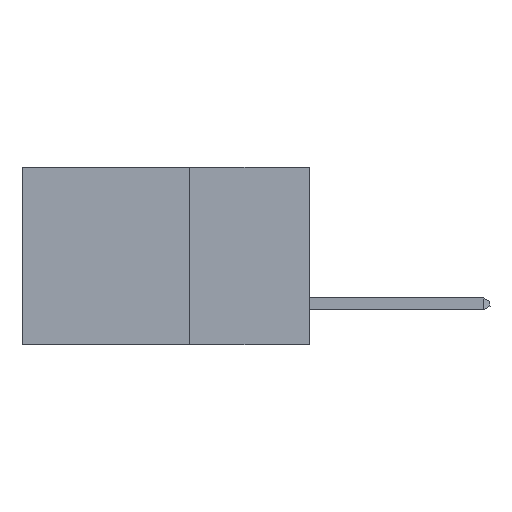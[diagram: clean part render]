
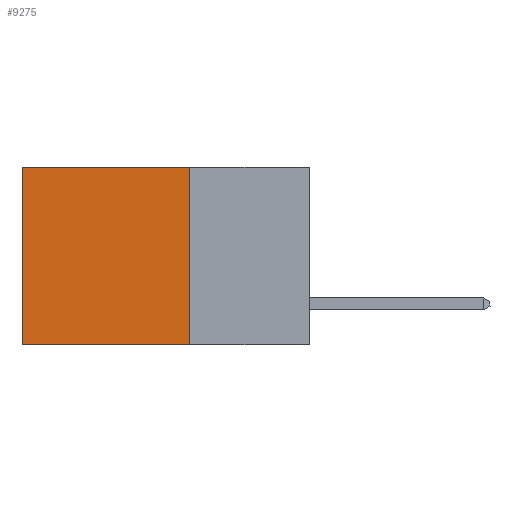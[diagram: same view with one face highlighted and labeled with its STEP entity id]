
A CAD part, left-side view. The second image highlights one B-rep face of the part: STEP entity #9275.
In plain terms, the highlighted planar face has unit normal (-1, 0, 0).
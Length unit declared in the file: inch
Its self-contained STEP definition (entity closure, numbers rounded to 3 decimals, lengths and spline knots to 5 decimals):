
#503 = EDGE_CURVE ( 'NONE', #8595, #10421, #12029, .T. ) ;
#1007 = EDGE_CURVE ( 'NONE', #14012, #10421, #18827, .T. ) ;
#1427 = CARTESIAN_POINT ( 'NONE',  ( 0.2875, 0.25, 0. ) ) ;
#1593 = EDGE_LOOP ( 'NONE', ( #12755, #6586, #19972, #16790 ) ) ;
#2520 = DIRECTION ( 'NONE',  ( 0., 1., 0. ) ) ;
#3064 = DIRECTION ( 'NONE',  ( 0., 0., -1. ) ) ;
#4185 = CARTESIAN_POINT ( 'NONE',  ( 0.2875, 0.6, -0.37 ) ) ;
#4750 = CARTESIAN_POINT ( 'NONE',  ( 0.2875, 0.25, 0. ) ) ;
#5290 = EDGE_CURVE ( 'NONE', #9811, #8595, #15781, .T. ) ;
#6255 = CARTESIAN_POINT ( 'NONE',  ( 0.2875, 0.25, -0.37 ) ) ;
#6586 = ORIENTED_EDGE ( 'NONE', *, *, #503, .F. ) ;
#7901 = PLANE ( 'NONE',  #13370 ) ;
#8172 = DIRECTION ( 'NONE',  ( 0., 0., -1. ) ) ;
#8595 = VERTEX_POINT ( 'NONE', #16961 ) ;
#9275 = ADVANCED_FACE ( 'NONE', ( #17598 ), #7901, .F. ) ;
#9811 = VERTEX_POINT ( 'NONE', #12326 ) ;
#10421 = VERTEX_POINT ( 'NONE', #4185 ) ;
#10518 = VECTOR ( 'NONE', #11832, 39.37008 ) ;
#11043 = VECTOR ( 'NONE', #2520, 39.37008 ) ;
#11109 = VECTOR ( 'NONE', #8172, 39.37008 ) ;
#11832 = DIRECTION ( 'NONE',  ( 0., 0., -1. ) ) ;
#12029 = LINE ( 'NONE', #6255, #11043 ) ;
#12326 = CARTESIAN_POINT ( 'NONE',  ( 0.2875, 0.25, 0. ) ) ;
#12685 = DIRECTION ( 'NONE',  ( 1., 0., 0. ) ) ;
#12755 = ORIENTED_EDGE ( 'NONE', *, *, #1007, .T. ) ;
#13370 = AXIS2_PLACEMENT_3D ( 'NONE', #1427, #12685, #3064 ) ;
#14012 = VERTEX_POINT ( 'NONE', #18884 ) ;
#14325 = VECTOR ( 'NONE', #20449, 39.37008 ) ;
#14833 = CARTESIAN_POINT ( 'NONE',  ( 0.2875, 0.6, 0. ) ) ;
#15781 = LINE ( 'NONE', #16043, #11109 ) ;
#16043 = CARTESIAN_POINT ( 'NONE',  ( 0.2875, 0.25, 0. ) ) ;
#16790 = ORIENTED_EDGE ( 'NONE', *, *, #19533, .T. ) ;
#16961 = CARTESIAN_POINT ( 'NONE',  ( 0.2875, 0.25, -0.37 ) ) ;
#17598 = FACE_OUTER_BOUND ( 'NONE', #1593, .T. ) ;
#18479 = LINE ( 'NONE', #4750, #14325 ) ;
#18827 = LINE ( 'NONE', #14833, #10518 ) ;
#18884 = CARTESIAN_POINT ( 'NONE',  ( 0.2875, 0.6, 0. ) ) ;
#19533 = EDGE_CURVE ( 'NONE', #9811, #14012, #18479, .T. ) ;
#19972 = ORIENTED_EDGE ( 'NONE', *, *, #5290, .F. ) ;
#20449 = DIRECTION ( 'NONE',  ( 0., 1., 0. ) ) ;
